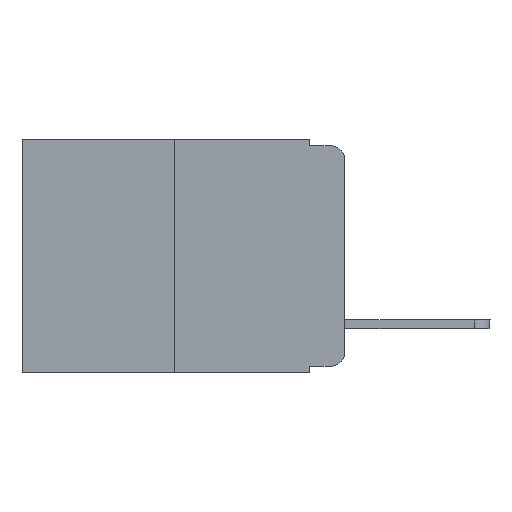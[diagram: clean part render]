
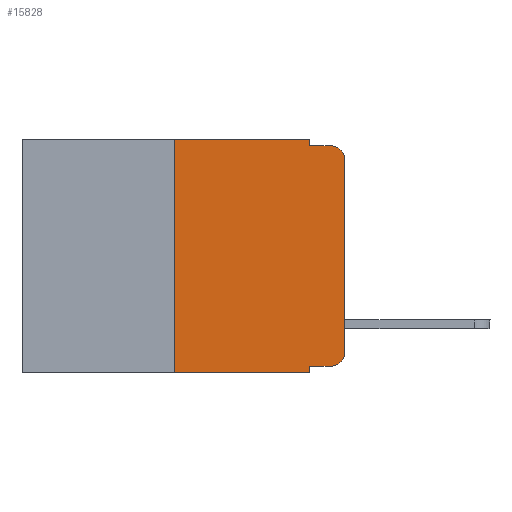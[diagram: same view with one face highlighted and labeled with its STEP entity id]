
A CAD part, left-side view. The second image highlights one B-rep face of the part: STEP entity #15828.
In plain terms, the highlighted planar face has unit normal (-1, 0, 0).
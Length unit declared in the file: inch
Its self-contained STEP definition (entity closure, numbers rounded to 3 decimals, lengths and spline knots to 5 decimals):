
#181 = LINE ( 'NONE', #7538, #15177 ) ;
#278 = CARTESIAN_POINT ( 'NONE',  ( 0., 0.25, 0. ) ) ;
#429 = EDGE_CURVE ( 'NONE', #7386, #2964, #17053, .T. ) ;
#708 = VERTEX_POINT ( 'NONE', #3731 ) ;
#723 = DIRECTION ( 'NONE',  ( -1., 0., 0. ) ) ;
#838 = ORIENTED_EDGE ( 'NONE', *, *, #15025, .T. ) ;
#1223 = CARTESIAN_POINT ( 'NONE',  ( 0., 0., -0.03 ) ) ;
#1314 = VERTEX_POINT ( 'NONE', #8015 ) ;
#1588 = CARTESIAN_POINT ( 'NONE',  ( 0., 0.051, -0.333 ) ) ;
#1683 = ORIENTED_EDGE ( 'NONE', *, *, #10396, .F. ) ;
#2019 = VECTOR ( 'NONE', #11580, 39.37008 ) ;
#2062 = VECTOR ( 'NONE', #12434, 39.37008 ) ;
#2250 = VERTEX_POINT ( 'NONE', #14392 ) ;
#2498 = CARTESIAN_POINT ( 'NONE',  ( 0., 0.473, 0. ) ) ;
#2580 = ORIENTED_EDGE ( 'NONE', *, *, #8896, .T. ) ;
#2618 = EDGE_LOOP ( 'NONE', ( #14834, #838, #6186, #9750, #12583, #3040, #11269, #1683, #2580, #4845 ) ) ;
#2911 = LINE ( 'NONE', #11523, #2019 ) ;
#2964 = VERTEX_POINT ( 'NONE', #9617 ) ;
#3040 = ORIENTED_EDGE ( 'NONE', *, *, #429, .F. ) ;
#3166 = CIRCLE ( 'NONE', #13312, 0.02 ) ;
#3230 = CARTESIAN_POINT ( 'NONE',  ( 0., 0.473, -0.343 ) ) ;
#3523 = CARTESIAN_POINT ( 'NONE',  ( 0., 0.02, -0.03 ) ) ;
#3731 = CARTESIAN_POINT ( 'NONE',  ( 0., 0.051, -0.333 ) ) ;
#4506 = VECTOR ( 'NONE', #15196, 39.37008 ) ;
#4641 = VERTEX_POINT ( 'NONE', #4891 ) ;
#4811 = LINE ( 'NONE', #8409, #10701 ) ;
#4845 = ORIENTED_EDGE ( 'NONE', *, *, #8797, .T. ) ;
#4891 = CARTESIAN_POINT ( 'NONE',  ( 0., 0., -0.313 ) ) ;
#4946 = VERTEX_POINT ( 'NONE', #5344 ) ;
#5117 = CARTESIAN_POINT ( 'NONE',  ( 0., 0.02, -0.01 ) ) ;
#5180 = EDGE_CURVE ( 'NONE', #7386, #1314, #16630, .T. ) ;
#5344 = CARTESIAN_POINT ( 'NONE',  ( 0., 0.02, -0.333 ) ) ;
#5864 = EDGE_CURVE ( 'NONE', #4641, #17051, #12952, .T. ) ;
#6186 = ORIENTED_EDGE ( 'NONE', *, *, #16339, .F. ) ;
#7386 = VERTEX_POINT ( 'NONE', #10874 ) ;
#7462 = DIRECTION ( 'NONE',  ( 0., -1., 0. ) ) ;
#7538 = CARTESIAN_POINT ( 'NONE',  ( 0., 0.473, 0. ) ) ;
#8015 = CARTESIAN_POINT ( 'NONE',  ( 0., 0.051, -0.343 ) ) ;
#8409 = CARTESIAN_POINT ( 'NONE',  ( 0., 0.051, -0.01 ) ) ;
#8639 = LINE ( 'NONE', #9350, #2062 ) ;
#8797 = EDGE_CURVE ( 'NONE', #4946, #4641, #3166, .T. ) ;
#8896 = EDGE_CURVE ( 'NONE', #708, #4946, #15447, .T. ) ;
#9029 = DIRECTION ( 'NONE',  ( 0., 0., 1. ) ) ;
#9350 = CARTESIAN_POINT ( 'NONE',  ( 0., 0.051, 0. ) ) ;
#9463 = AXIS2_PLACEMENT_3D ( 'NONE', #3523, #13716, #15360 ) ;
#9521 = VERTEX_POINT ( 'NONE', #5117 ) ;
#9617 = CARTESIAN_POINT ( 'NONE',  ( 0., 0.25, 0. ) ) ;
#9750 = ORIENTED_EDGE ( 'NONE', *, *, #17414, .F. ) ;
#9764 = VECTOR ( 'NONE', #17803, 39.37008 ) ;
#9829 = DIRECTION ( 'NONE',  ( 0., 0., -1. ) ) ;
#9981 = DIRECTION ( 'NONE',  ( 0., -1., 0. ) ) ;
#10396 = EDGE_CURVE ( 'NONE', #708, #1314, #2911, .T. ) ;
#10701 = VECTOR ( 'NONE', #9981, 39.37008 ) ;
#10874 = CARTESIAN_POINT ( 'NONE',  ( 0., 0.25, -0.343 ) ) ;
#11269 = ORIENTED_EDGE ( 'NONE', *, *, #5180, .T. ) ;
#11523 = CARTESIAN_POINT ( 'NONE',  ( 0., 0.051, 0. ) ) ;
#11580 = DIRECTION ( 'NONE',  ( 0., 0., -1. ) ) ;
#12434 = DIRECTION ( 'NONE',  ( 0., 0., -1. ) ) ;
#12578 = FACE_OUTER_BOUND ( 'NONE', #2618, .T. ) ;
#12583 = ORIENTED_EDGE ( 'NONE', *, *, #14268, .F. ) ;
#12652 = DIRECTION ( 'NONE',  ( 1., 0., 0. ) ) ;
#12952 = LINE ( 'NONE', #17845, #17077 ) ;
#13312 = AXIS2_PLACEMENT_3D ( 'NONE', #18002, #723, #15326 ) ;
#13528 = CIRCLE ( 'NONE', #9463, 0.02 ) ;
#13716 = DIRECTION ( 'NONE',  ( -1., 0., 0. ) ) ;
#14268 = EDGE_CURVE ( 'NONE', #2964, #2250, #181, .T. ) ;
#14269 = AXIS2_PLACEMENT_3D ( 'NONE', #2498, #12652, #9829 ) ;
#14392 = CARTESIAN_POINT ( 'NONE',  ( 0., 0.051, 0. ) ) ;
#14706 = CARTESIAN_POINT ( 'NONE',  ( 0., 0.051, -0.01 ) ) ;
#14834 = ORIENTED_EDGE ( 'NONE', *, *, #5864, .T. ) ;
#15025 = EDGE_CURVE ( 'NONE', #17051, #9521, #13528, .T. ) ;
#15177 = VECTOR ( 'NONE', #16229, 39.37008 ) ;
#15196 = DIRECTION ( 'NONE',  ( 0., 0., 1. ) ) ;
#15326 = DIRECTION ( 'NONE',  ( 0., 0., -1. ) ) ;
#15360 = DIRECTION ( 'NONE',  ( 0., 0., -1. ) ) ;
#15447 = LINE ( 'NONE', #1588, #17743 ) ;
#15828 = ADVANCED_FACE ( 'NONE', ( #12578 ), #17192, .F. ) ;
#16229 = DIRECTION ( 'NONE',  ( 0., -1., 0. ) ) ;
#16339 = EDGE_CURVE ( 'NONE', #16493, #9521, #4811, .T. ) ;
#16493 = VERTEX_POINT ( 'NONE', #14706 ) ;
#16630 = LINE ( 'NONE', #3230, #9764 ) ;
#17051 = VERTEX_POINT ( 'NONE', #1223 ) ;
#17053 = LINE ( 'NONE', #278, #4506 ) ;
#17077 = VECTOR ( 'NONE', #9029, 39.37008 ) ;
#17192 = PLANE ( 'NONE',  #14269 ) ;
#17414 = EDGE_CURVE ( 'NONE', #2250, #16493, #8639, .T. ) ;
#17743 = VECTOR ( 'NONE', #7462, 39.37008 ) ;
#17803 = DIRECTION ( 'NONE',  ( 0., -1., 0. ) ) ;
#17845 = CARTESIAN_POINT ( 'NONE',  ( 0., 0., 0. ) ) ;
#18002 = CARTESIAN_POINT ( 'NONE',  ( 0., 0.02, -0.313 ) ) ;
